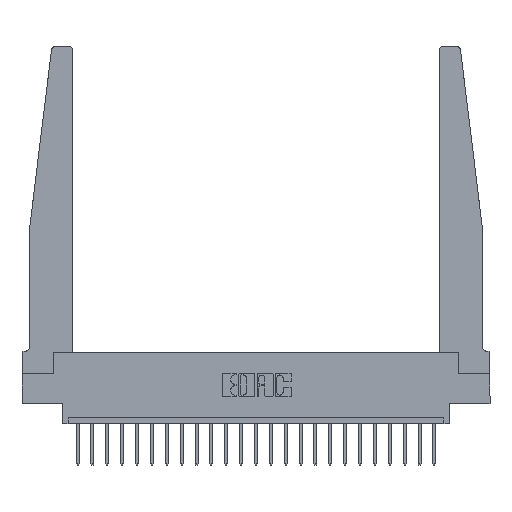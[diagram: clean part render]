
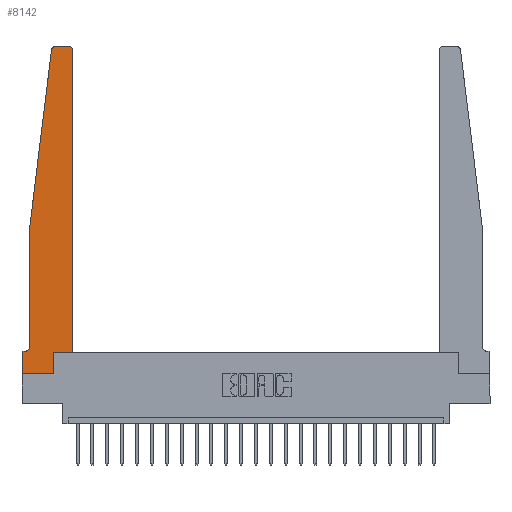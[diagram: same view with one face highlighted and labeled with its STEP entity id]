
A CAD part, top view. The second image highlights one B-rep face of the part: STEP entity #8142.
In plain terms, the highlighted planar face has unit normal (0, 0, 1).
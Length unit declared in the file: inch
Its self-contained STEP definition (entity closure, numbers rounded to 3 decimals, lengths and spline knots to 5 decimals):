
#320 = VERTEX_POINT ( 'NONE', #19247 ) ;
#428 = VERTEX_POINT ( 'NONE', #1119 ) ;
#799 = PLANE ( 'NONE',  #22800 ) ;
#1034 = FACE_OUTER_BOUND ( 'NONE', #6090, .T. ) ;
#1109 = DIRECTION ( 'NONE',  ( 1., 0., 0. ) ) ;
#1119 = CARTESIAN_POINT ( 'NONE',  ( 0.24675, 2.72367, 0.37 ) ) ;
#1268 = EDGE_CURVE ( 'NONE', #320, #13168, #11481, .T. ) ;
#1538 = LINE ( 'NONE', #18595, #1689 ) ;
#1677 = CARTESIAN_POINT ( 'NONE',  ( 0.425, 2.72, 0.37 ) ) ;
#1689 = VECTOR ( 'NONE', #6091, 39.37008 ) ;
#1927 = DIRECTION ( 'NONE',  ( 1., 0., 0. ) ) ;
#1930 = DIRECTION ( 'NONE',  ( 0., -1., 0. ) ) ;
#2043 = DIRECTION ( 'NONE',  ( 0., 0., 1. ) ) ;
#2410 = EDGE_CURVE ( 'NONE', #20263, #12114, #16308, .T. ) ;
#2779 = CARTESIAN_POINT ( 'NONE',  ( 0., 0.1875, 0.37 ) ) ;
#2805 = DIRECTION ( 'NONE',  ( 1., 0., 0. ) ) ;
#2963 = CARTESIAN_POINT ( 'NONE',  ( 0.065, 1.25, 0.37 ) ) ;
#3370 = DIRECTION ( 'NONE',  ( 0., -1., 0. ) ) ;
#3606 = DIRECTION ( 'NONE',  ( 0., 0., -1. ) ) ;
#3622 = CARTESIAN_POINT ( 'NONE',  ( 0.27653, 2.72, 0.37 ) ) ;
#3724 = CARTESIAN_POINT ( 'NONE',  ( 0.015, 0.2375, 0.37 ) ) ;
#4797 = LINE ( 'NONE', #19412, #13934 ) ;
#4892 = AXIS2_PLACEMENT_3D ( 'NONE', #3622, #19441, #16160 ) ;
#4951 = CARTESIAN_POINT ( 'NONE',  ( 0.425, 0.18, 0.37 ) ) ;
#5110 = EDGE_CURVE ( 'NONE', #16195, #320, #6148, .T. ) ;
#5363 = DIRECTION ( 'NONE',  ( 0., 1., 0. ) ) ;
#5916 = CARTESIAN_POINT ( 'NONE',  ( 0.25, 2.75, 0.37 ) ) ;
#6090 = EDGE_LOOP ( 'NONE', ( #10025, #9359, #17754, #14223, #12168, #10608, #16096, #7473, #19573, #16450, #22443, #14349 ) ) ;
#6091 = DIRECTION ( 'NONE',  ( -0.122, -0.992, 0. ) ) ;
#6148 = LINE ( 'NONE', #17143, #10533 ) ;
#6217 = DIRECTION ( 'NONE',  ( 0., 1., 0. ) ) ;
#6300 = CARTESIAN_POINT ( 'NONE',  ( 0.065, 0.2375, 0.37 ) ) ;
#6511 = EDGE_CURVE ( 'NONE', #13168, #22661, #9503, .T. ) ;
#6854 = EDGE_CURVE ( 'NONE', #18561, #17907, #21965, .T. ) ;
#6912 = DIRECTION ( 'NONE',  ( -1., 0., 0. ) ) ;
#6938 = VECTOR ( 'NONE', #5363, 39.37008 ) ;
#7124 = CIRCLE ( 'NONE', #4892, 0.03 ) ;
#7223 = LINE ( 'NONE', #14258, #6938 ) ;
#7406 = CARTESIAN_POINT ( 'NONE',  ( 0.065, 0.1875, 0.37 ) ) ;
#7473 = ORIENTED_EDGE ( 'NONE', *, *, #5110, .T. ) ;
#7923 = EDGE_CURVE ( 'NONE', #11273, #16195, #4797, .T. ) ;
#7942 = DIRECTION ( 'NONE',  ( 0., 0., 1. ) ) ;
#8142 = ADVANCED_FACE ( 'NONE', ( #1034 ), #799, .T. ) ;
#9056 = VECTOR ( 'NONE', #1930, 39.37008 ) ;
#9204 = CARTESIAN_POINT ( 'NONE',  ( 0.395, 2.72, 0.37 ) ) ;
#9359 = ORIENTED_EDGE ( 'NONE', *, *, #12538, .T. ) ;
#9503 = LINE ( 'NONE', #18835, #18592 ) ;
#9830 = CARTESIAN_POINT ( 'NONE',  ( 0.395, 2.75, 0.37 ) ) ;
#10025 = ORIENTED_EDGE ( 'NONE', *, *, #6854, .T. ) ;
#10261 = VECTOR ( 'NONE', #21711, 39.37008 ) ;
#10505 = EDGE_CURVE ( 'NONE', #14868, #18561, #13856, .T. ) ;
#10533 = VECTOR ( 'NONE', #1109, 39.37008 ) ;
#10608 = ORIENTED_EDGE ( 'NONE', *, *, #16427, .T. ) ;
#11273 = VERTEX_POINT ( 'NONE', #14839 ) ;
#11481 = LINE ( 'NONE', #22486, #12075 ) ;
#12075 = VECTOR ( 'NONE', #6217, 39.37008 ) ;
#12114 = VERTEX_POINT ( 'NONE', #18051 ) ;
#12168 = ORIENTED_EDGE ( 'NONE', *, *, #2410, .T. ) ;
#12538 = EDGE_CURVE ( 'NONE', #17907, #428, #7124, .T. ) ;
#12699 = CARTESIAN_POINT ( 'NONE',  ( 0., 0., 0.37 ) ) ;
#12802 = CARTESIAN_POINT ( 'NONE',  ( 0.27653, 2.75, 0.37 ) ) ;
#13072 = DIRECTION ( 'NONE',  ( -1., 0., 0. ) ) ;
#13168 = VERTEX_POINT ( 'NONE', #18325 ) ;
#13856 = CIRCLE ( 'NONE', #20594, 0.03 ) ;
#13934 = VECTOR ( 'NONE', #3370, 39.37008 ) ;
#14223 = ORIENTED_EDGE ( 'NONE', *, *, #14437, .T. ) ;
#14258 = CARTESIAN_POINT ( 'NONE',  ( 0.425, 0.18, 0.37 ) ) ;
#14349 = ORIENTED_EDGE ( 'NONE', *, *, #10505, .T. ) ;
#14437 = EDGE_CURVE ( 'NONE', #22550, #20263, #15762, .T. ) ;
#14839 = CARTESIAN_POINT ( 'NONE',  ( 0., 0.1875, 0.37 ) ) ;
#14868 = VERTEX_POINT ( 'NONE', #1677 ) ;
#15078 = DIRECTION ( 'NONE',  ( 1., 0., 0. ) ) ;
#15762 = LINE ( 'NONE', #22904, #9056 ) ;
#16096 = ORIENTED_EDGE ( 'NONE', *, *, #7923, .T. ) ;
#16160 = DIRECTION ( 'NONE',  ( 1., 0., 0. ) ) ;
#16195 = VERTEX_POINT ( 'NONE', #12699 ) ;
#16308 = CIRCLE ( 'NONE', #17793, 0.05 ) ;
#16427 = EDGE_CURVE ( 'NONE', #12114, #11273, #16549, .T. ) ;
#16450 = ORIENTED_EDGE ( 'NONE', *, *, #6511, .T. ) ;
#16549 = LINE ( 'NONE', #7406, #10261 ) ;
#17143 = CARTESIAN_POINT ( 'NONE',  ( 0., 0., 0.37 ) ) ;
#17754 = ORIENTED_EDGE ( 'NONE', *, *, #19590, .T. ) ;
#17793 = AXIS2_PLACEMENT_3D ( 'NONE', #3724, #3606, #6912 ) ;
#17907 = VERTEX_POINT ( 'NONE', #12802 ) ;
#18051 = CARTESIAN_POINT ( 'NONE',  ( 0.015, 0.1875, 0.37 ) ) ;
#18325 = CARTESIAN_POINT ( 'NONE',  ( 0.2605, 0.18, 0.37 ) ) ;
#18561 = VERTEX_POINT ( 'NONE', #9830 ) ;
#18592 = VECTOR ( 'NONE', #2805, 39.37008 ) ;
#18595 = CARTESIAN_POINT ( 'NONE',  ( 0.065, 1.25, 0.37 ) ) ;
#18835 = CARTESIAN_POINT ( 'NONE',  ( 0.425, 0.18, 0.37 ) ) ;
#19247 = CARTESIAN_POINT ( 'NONE',  ( 0.2605, 0., 0.37 ) ) ;
#19412 = CARTESIAN_POINT ( 'NONE',  ( 0., 0., 0.37 ) ) ;
#19441 = DIRECTION ( 'NONE',  ( 0., 0., 1. ) ) ;
#19573 = ORIENTED_EDGE ( 'NONE', *, *, #1268, .T. ) ;
#19590 = EDGE_CURVE ( 'NONE', #428, #22550, #1538, .T. ) ;
#20033 = EDGE_CURVE ( 'NONE', #22661, #14868, #7223, .T. ) ;
#20263 = VERTEX_POINT ( 'NONE', #6300 ) ;
#20594 = AXIS2_PLACEMENT_3D ( 'NONE', #9204, #2043, #1927 ) ;
#20683 = VECTOR ( 'NONE', #13072, 39.37008 ) ;
#21711 = DIRECTION ( 'NONE',  ( -1., 0., 0. ) ) ;
#21965 = LINE ( 'NONE', #5916, #20683 ) ;
#22443 = ORIENTED_EDGE ( 'NONE', *, *, #20033, .T. ) ;
#22486 = CARTESIAN_POINT ( 'NONE',  ( 0.2605, 0.18, 0.37 ) ) ;
#22550 = VERTEX_POINT ( 'NONE', #2963 ) ;
#22661 = VERTEX_POINT ( 'NONE', #4951 ) ;
#22800 = AXIS2_PLACEMENT_3D ( 'NONE', #2779, #7942, #15078 ) ;
#22904 = CARTESIAN_POINT ( 'NONE',  ( 0.065, 1.25, 0.37 ) ) ;
